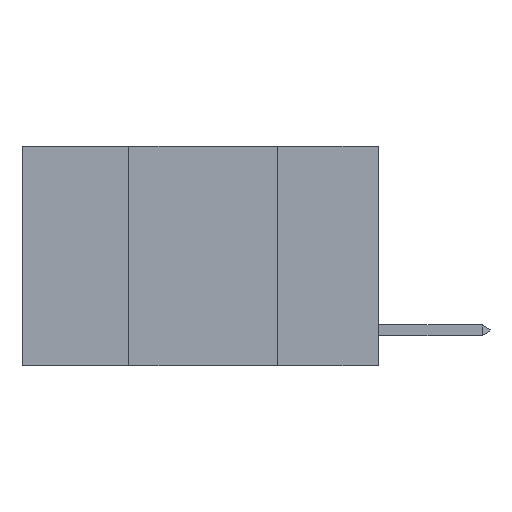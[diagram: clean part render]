
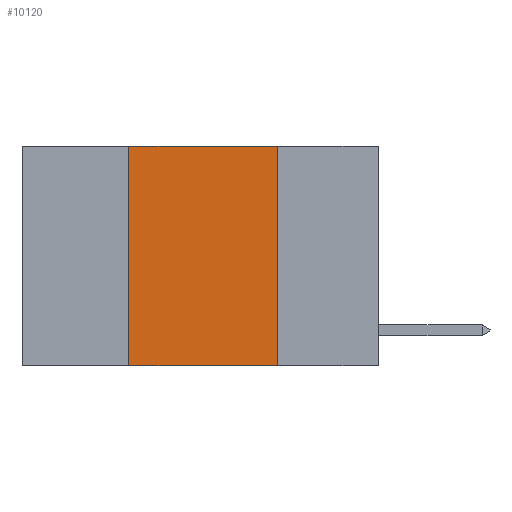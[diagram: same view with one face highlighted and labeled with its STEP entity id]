
A CAD part, left-side view. The second image highlights one B-rep face of the part: STEP entity #10120.
In plain terms, the highlighted planar face has unit normal (-1, 0, 0).
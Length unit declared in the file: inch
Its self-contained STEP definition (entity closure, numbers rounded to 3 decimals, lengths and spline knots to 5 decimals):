
#484 = EDGE_CURVE ( 'NONE', #14300, #1944, #3519, .T. ) ;
#1562 = VECTOR ( 'NONE', #12723, 39.37008 ) ;
#1944 = VERTEX_POINT ( 'NONE', #2315 ) ;
#2034 = VECTOR ( 'NONE', #19329, 39.37008 ) ;
#2097 = EDGE_LOOP ( 'NONE', ( #8673, #6248, #22284, #11978 ) ) ;
#2176 = VERTEX_POINT ( 'NONE', #12178 ) ;
#2246 = PLANE ( 'NONE',  #23076 ) ;
#2315 = CARTESIAN_POINT ( 'NONE',  ( 0., 0.17, 0. ) ) ;
#3519 = LINE ( 'NONE', #5223, #2034 ) ;
#5223 = CARTESIAN_POINT ( 'NONE',  ( 0., 0.6, 0. ) ) ;
#6248 = ORIENTED_EDGE ( 'NONE', *, *, #484, .F. ) ;
#6283 = DIRECTION ( 'NONE',  ( 0., 0., -1. ) ) ;
#8271 = DIRECTION ( 'NONE',  ( 1., 0., 0. ) ) ;
#8673 = ORIENTED_EDGE ( 'NONE', *, *, #16243, .F. ) ;
#9877 = CARTESIAN_POINT ( 'NONE',  ( 0., 0.17, -0.37 ) ) ;
#9887 = DIRECTION ( 'NONE',  ( 0., -1., 0. ) ) ;
#10120 = ADVANCED_FACE ( 'NONE', ( #20132 ), #2246, .F. ) ;
#11824 = LINE ( 'NONE', #19809, #18293 ) ;
#11978 = ORIENTED_EDGE ( 'NONE', *, *, #18169, .T. ) ;
#12178 = CARTESIAN_POINT ( 'NONE',  ( 0., 0.42, -0.37 ) ) ;
#12723 = DIRECTION ( 'NONE',  ( 0., 0., 1. ) ) ;
#13345 = CARTESIAN_POINT ( 'NONE',  ( 0., 0.17, 0. ) ) ;
#13588 = DIRECTION ( 'NONE',  ( 0., 0., -1. ) ) ;
#14300 = VERTEX_POINT ( 'NONE', #20260 ) ;
#14460 = VECTOR ( 'NONE', #13588, 39.37008 ) ;
#14684 = CARTESIAN_POINT ( 'NONE',  ( 0., 0.42, 0. ) ) ;
#16243 = EDGE_CURVE ( 'NONE', #1944, #16809, #25034, .T. ) ;
#16809 = VERTEX_POINT ( 'NONE', #9877 ) ;
#18147 = CARTESIAN_POINT ( 'NONE',  ( 0., 0.6, 0. ) ) ;
#18169 = EDGE_CURVE ( 'NONE', #2176, #16809, #11824, .T. ) ;
#18293 = VECTOR ( 'NONE', #9887, 39.37008 ) ;
#18470 = LINE ( 'NONE', #14684, #1562 ) ;
#19329 = DIRECTION ( 'NONE',  ( 0., -1., 0. ) ) ;
#19809 = CARTESIAN_POINT ( 'NONE',  ( 0., 0.6, -0.37 ) ) ;
#20132 = FACE_OUTER_BOUND ( 'NONE', #2097, .T. ) ;
#20260 = CARTESIAN_POINT ( 'NONE',  ( 0., 0.42, 0. ) ) ;
#20808 = EDGE_CURVE ( 'NONE', #2176, #14300, #18470, .T. ) ;
#22284 = ORIENTED_EDGE ( 'NONE', *, *, #20808, .F. ) ;
#23076 = AXIS2_PLACEMENT_3D ( 'NONE', #18147, #8271, #6283 ) ;
#25034 = LINE ( 'NONE', #13345, #14460 ) ;
